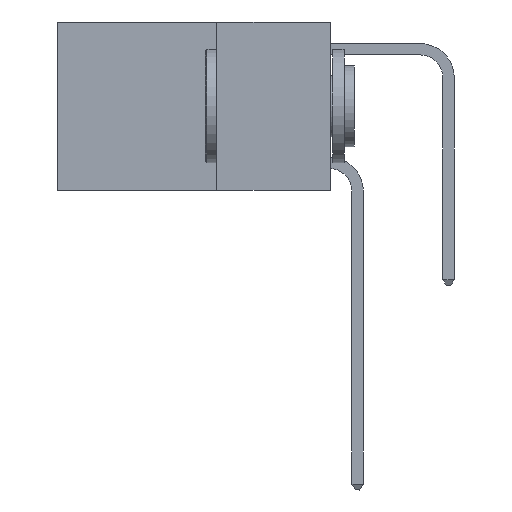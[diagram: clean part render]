
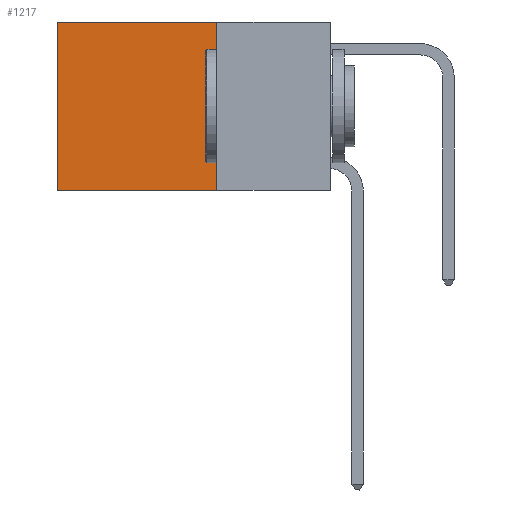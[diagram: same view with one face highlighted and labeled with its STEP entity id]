
A CAD part, left-side view. The second image highlights one B-rep face of the part: STEP entity #1217.
In plain terms, the highlighted planar face has unit normal (-1, 0, 0).
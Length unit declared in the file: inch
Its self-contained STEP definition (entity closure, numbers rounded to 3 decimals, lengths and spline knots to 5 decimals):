
#332 = EDGE_CURVE ( 'NONE', #7809, #4975, #7859, .T. ) ;
#540 = CARTESIAN_POINT ( 'NONE',  ( 0.2625, 0.25, -0.37 ) ) ;
#621 = VECTOR ( 'NONE', #8332, 39.37008 ) ;
#942 = CARTESIAN_POINT ( 'NONE',  ( 0.2625, 0.6, 0. ) ) ;
#1109 = VECTOR ( 'NONE', #9349, 39.37008 ) ;
#1217 = ADVANCED_FACE ( 'NONE', ( #5555 ), #6735, .F. ) ;
#1587 = CARTESIAN_POINT ( 'NONE',  ( 0.2625, 0.25, 0. ) ) ;
#1810 = DIRECTION ( 'NONE',  ( 0., 0., -1. ) ) ;
#2394 = ORIENTED_EDGE ( 'NONE', *, *, #11729, .T. ) ;
#2699 = LINE ( 'NONE', #4024, #13571 ) ;
#2722 = DIRECTION ( 'NONE',  ( 0., 0., -1. ) ) ;
#3414 = ORIENTED_EDGE ( 'NONE', *, *, #8527, .F. ) ;
#4024 = CARTESIAN_POINT ( 'NONE',  ( 0.2625, 0.6, 0. ) ) ;
#4062 = LINE ( 'NONE', #8273, #1109 ) ;
#4975 = VERTEX_POINT ( 'NONE', #942 ) ;
#5555 = FACE_OUTER_BOUND ( 'NONE', #13713, .T. ) ;
#5867 = LINE ( 'NONE', #1587, #11145 ) ;
#6548 = CARTESIAN_POINT ( 'NONE',  ( 0.2625, 0.25, 0. ) ) ;
#6735 = PLANE ( 'NONE',  #13142 ) ;
#7809 = VERTEX_POINT ( 'NONE', #6548 ) ;
#7859 = LINE ( 'NONE', #9255, #621 ) ;
#8174 = VERTEX_POINT ( 'NONE', #10941 ) ;
#8273 = CARTESIAN_POINT ( 'NONE',  ( 0.2625, 0.25, -0.37 ) ) ;
#8332 = DIRECTION ( 'NONE',  ( 0., 1., 0. ) ) ;
#8527 = EDGE_CURVE ( 'NONE', #11617, #8174, #4062, .T. ) ;
#9103 = EDGE_CURVE ( 'NONE', #7809, #11617, #5867, .T. ) ;
#9136 = ORIENTED_EDGE ( 'NONE', *, *, #9103, .F. ) ;
#9255 = CARTESIAN_POINT ( 'NONE',  ( 0.2625, 0.25, 0. ) ) ;
#9349 = DIRECTION ( 'NONE',  ( 0., 1., 0. ) ) ;
#10767 = DIRECTION ( 'NONE',  ( 0., 0., -1. ) ) ;
#10941 = CARTESIAN_POINT ( 'NONE',  ( 0.2625, 0.6, -0.37 ) ) ;
#11145 = VECTOR ( 'NONE', #2722, 39.37008 ) ;
#11617 = VERTEX_POINT ( 'NONE', #540 ) ;
#11729 = EDGE_CURVE ( 'NONE', #4975, #8174, #2699, .T. ) ;
#12455 = DIRECTION ( 'NONE',  ( 1., 0., 0. ) ) ;
#12738 = CARTESIAN_POINT ( 'NONE',  ( 0.2625, 0.25, 0. ) ) ;
#12934 = ORIENTED_EDGE ( 'NONE', *, *, #332, .T. ) ;
#13142 = AXIS2_PLACEMENT_3D ( 'NONE', #12738, #12455, #10767 ) ;
#13571 = VECTOR ( 'NONE', #1810, 39.37008 ) ;
#13713 = EDGE_LOOP ( 'NONE', ( #2394, #3414, #9136, #12934 ) ) ;
